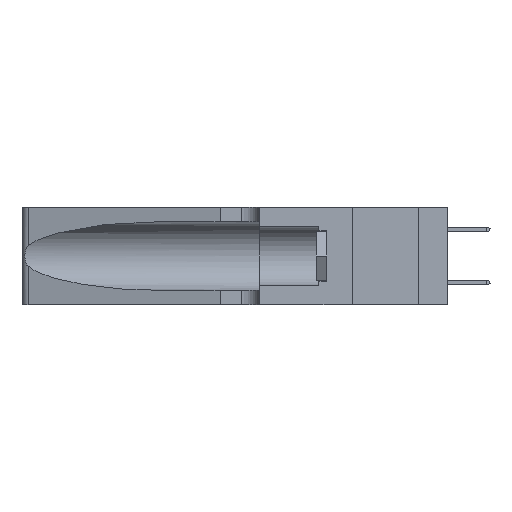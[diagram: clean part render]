
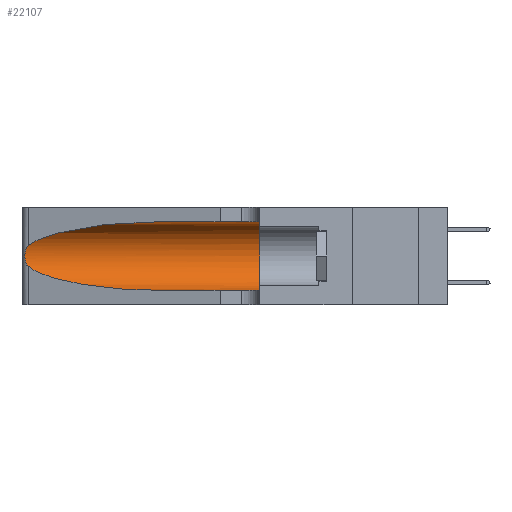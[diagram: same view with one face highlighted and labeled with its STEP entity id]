
A CAD part, left-side view. The second image highlights one B-rep face of the part: STEP entity #22107.
In plain terms, the highlighted cylindrical face has radius 3.308 mm (diameter 6.617 mm), a partial arc.
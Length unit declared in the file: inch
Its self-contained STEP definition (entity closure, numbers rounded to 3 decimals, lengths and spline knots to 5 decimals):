
#160 = DIRECTION ( 'NONE',  ( 0., -1., 0. ) ) ;
#1011 = CARTESIAN_POINT ( 'NONE',  ( 0.2373, 1.15595, 0.28018 ) ) ;
#1536 = CARTESIAN_POINT ( 'NONE',  ( 0.25555, 1.22993, 0.14849 ) ) ;
#2015 = VECTOR ( 'NONE', #15387, 39.37008 ) ;
#2053 =( BOUNDED_CURVE ( )  B_SPLINE_CURVE ( 3, ( #7423, #20732, #25265, #11855 ),
 .UNSPECIFIED., .F., .T. ) 
 B_SPLINE_CURVE_WITH_KNOTS ( ( 4, 4 ),
 ( 3.44316, 4.71239 ),
 .UNSPECIFIED. ) 
 CURVE ( )  GEOMETRIC_REPRESENTATION_ITEM ( )  RATIONAL_B_SPLINE_CURVE ( ( 1., 0.87, 0.87, 1. ) ) 
 REPRESENTATION_ITEM ( '' )  );
#2073 = ORIENTED_EDGE ( 'NONE', *, *, #3785, .T. ) ;
#2371 = CARTESIAN_POINT ( 'NONE',  ( 0.1305, 1.61858, 0.185 ) ) ;
#2770 = EDGE_LOOP ( 'NONE', ( #11456, #2073, #17184, #17482, #23550, #20937 ) ) ;
#2968 = EDGE_CURVE ( 'NONE', #18010, #5449, #4197, .T. ) ;
#3785 = EDGE_CURVE ( 'NONE', #5449, #22095, #9322, .T. ) ;
#4197 =( BOUNDED_CURVE ( )  B_SPLINE_CURVE ( 3, ( #20998, #16477, #1011, #7666 ),
 .UNSPECIFIED., .F., .T. ) 
 B_SPLINE_CURVE_WITH_KNOTS ( ( 4, 4 ),
 ( 1.5708, 2.84003 ),
 .UNSPECIFIED. ) 
 CURVE ( )  GEOMETRIC_REPRESENTATION_ITEM ( )  RATIONAL_B_SPLINE_CURVE ( ( 1., 0.87, 0.87, 1. ) ) 
 REPRESENTATION_ITEM ( '' )  );
#4652 = AXIS2_PLACEMENT_3D ( 'NONE', #2371, #160, #20024 ) ;
#5075 = CARTESIAN_POINT ( 'NONE',  ( 0.1305, 0.72297, 0.05475 ) ) ;
#5449 = VERTEX_POINT ( 'NONE', #8031 ) ;
#5869 = CARTESIAN_POINT ( 'NONE',  ( 0.25787, 1.23484, 0.2124 ) ) ;
#5872 = DIRECTION ( 'NONE',  ( 0., 1., 0. ) ) ;
#5982 = CYLINDRICAL_SURFACE ( 'NONE', #4652, 0.13025 ) ;
#6681 = FACE_OUTER_BOUND ( 'NONE', #2770, .T. ) ;
#7423 = CARTESIAN_POINT ( 'NONE',  ( 0.25487, 1.22718, 0.14631 ) ) ;
#7666 = CARTESIAN_POINT ( 'NONE',  ( 0.25487, 1.22718, 0.22369 ) ) ;
#8031 = CARTESIAN_POINT ( 'NONE',  ( 0.25487, 1.22718, 0.22369 ) ) ;
#8093 = CARTESIAN_POINT ( 'NONE',  ( 0.26018, 1.23835, 0.19895 ) ) ;
#9082 = CARTESIAN_POINT ( 'NONE',  ( 0.1305, 0.35, 0.05475 ) ) ;
#9322 = B_SPLINE_CURVE_WITH_KNOTS ( 'NONE', 3,
 ( #21346, #16928, #19178, #5869, #21433, #8093, #23706, #10306, #25969, #12534, #28206, #14743, #1536, #17022 ),
 .UNSPECIFIED., .F., .F.,
 ( 4, 2, 2, 2, 2, 2, 4 ),
 ( 0., 0.00027, 0.00053, 0.00107, 0.0016, 0.00187, 0.00214 ),
 .UNSPECIFIED. ) ;
#9994 = CARTESIAN_POINT ( 'NONE',  ( 0.1305, 0.72297, 0.31525 ) ) ;
#10306 = CARTESIAN_POINT ( 'NONE',  ( 0.26075, 1.23896, 0.178 ) ) ;
#11047 = VECTOR ( 'NONE', #20623, 39.37008 ) ;
#11456 = ORIENTED_EDGE ( 'NONE', *, *, #2968, .T. ) ;
#11855 = CARTESIAN_POINT ( 'NONE',  ( 0.1305, 0.72297, 0.05475 ) ) ;
#12534 = CARTESIAN_POINT ( 'NONE',  ( 0.25856, 1.23593, 0.16098 ) ) ;
#13800 = EDGE_CURVE ( 'NONE', #19852, #14980, #25724, .T. ) ;
#14743 = CARTESIAN_POINT ( 'NONE',  ( 0.25639, 1.23186, 0.15144 ) ) ;
#14980 = VERTEX_POINT ( 'NONE', #9082 ) ;
#15387 = DIRECTION ( 'NONE',  ( 0., -1., 0. ) ) ;
#15539 = LINE ( 'NONE', #16109, #11047 ) ;
#15881 = AXIS2_PLACEMENT_3D ( 'NONE', #19182, #5872, #21437 ) ;
#16109 = CARTESIAN_POINT ( 'NONE',  ( 0.1305, 1.61858, 0.31525 ) ) ;
#16477 = CARTESIAN_POINT ( 'NONE',  ( 0.18966, 0.96281, 0.31525 ) ) ;
#16928 = CARTESIAN_POINT ( 'NONE',  ( 0.25555, 1.22994, 0.2215 ) ) ;
#17022 = CARTESIAN_POINT ( 'NONE',  ( 0.25487, 1.22718, 0.14631 ) ) ;
#17184 = ORIENTED_EDGE ( 'NONE', *, *, #17908, .T. ) ;
#17271 = EDGE_CURVE ( 'NONE', #17614, #14980, #28707, .T. ) ;
#17482 = ORIENTED_EDGE ( 'NONE', *, *, #13800, .T. ) ;
#17614 = VERTEX_POINT ( 'NONE', #19767 ) ;
#17908 = EDGE_CURVE ( 'NONE', #22095, #19852, #2053, .T. ) ;
#18010 = VERTEX_POINT ( 'NONE', #9994 ) ;
#19178 = CARTESIAN_POINT ( 'NONE',  ( 0.25639, 1.23184, 0.21858 ) ) ;
#19182 = CARTESIAN_POINT ( 'NONE',  ( 0.1305, 0.35, 0.185 ) ) ;
#19767 = CARTESIAN_POINT ( 'NONE',  ( 0.1305, 0.35, 0.31525 ) ) ;
#19852 = VERTEX_POINT ( 'NONE', #5075 ) ;
#20024 = DIRECTION ( 'NONE',  ( 0., 0., -1. ) ) ;
#20623 = DIRECTION ( 'NONE',  ( 0., -1., 0. ) ) ;
#20732 = CARTESIAN_POINT ( 'NONE',  ( 0.2373, 1.15595, 0.08982 ) ) ;
#20937 = ORIENTED_EDGE ( 'NONE', *, *, #24008, .F. ) ;
#20998 = CARTESIAN_POINT ( 'NONE',  ( 0.1305, 0.72297, 0.31525 ) ) ;
#21346 = CARTESIAN_POINT ( 'NONE',  ( 0.25487, 1.22718, 0.22369 ) ) ;
#21433 = CARTESIAN_POINT ( 'NONE',  ( 0.25854, 1.2359, 0.20912 ) ) ;
#21437 = DIRECTION ( 'NONE',  ( 0., 0., 1. ) ) ;
#22095 = VERTEX_POINT ( 'NONE', #26832 ) ;
#22107 = ADVANCED_FACE ( 'NONE', ( #6681 ), #5982, .F. ) ;
#23550 = ORIENTED_EDGE ( 'NONE', *, *, #17271, .F. ) ;
#23706 = CARTESIAN_POINT ( 'NONE',  ( 0.26075, 1.23896, 0.19203 ) ) ;
#24008 = EDGE_CURVE ( 'NONE', #18010, #17614, #15539, .T. ) ;
#24352 = CARTESIAN_POINT ( 'NONE',  ( 0.1305, 1.61858, 0.05475 ) ) ;
#25265 = CARTESIAN_POINT ( 'NONE',  ( 0.18966, 0.96281, 0.05475 ) ) ;
#25724 = LINE ( 'NONE', #24352, #2015 ) ;
#25969 = CARTESIAN_POINT ( 'NONE',  ( 0.26017, 1.23833, 0.17102 ) ) ;
#26832 = CARTESIAN_POINT ( 'NONE',  ( 0.25487, 1.22718, 0.14631 ) ) ;
#28206 = CARTESIAN_POINT ( 'NONE',  ( 0.25789, 1.23486, 0.15765 ) ) ;
#28707 = CIRCLE ( 'NONE', #15881, 0.13025 ) ;
